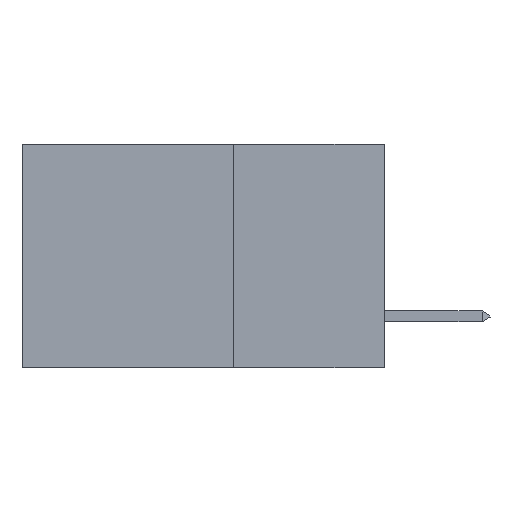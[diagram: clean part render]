
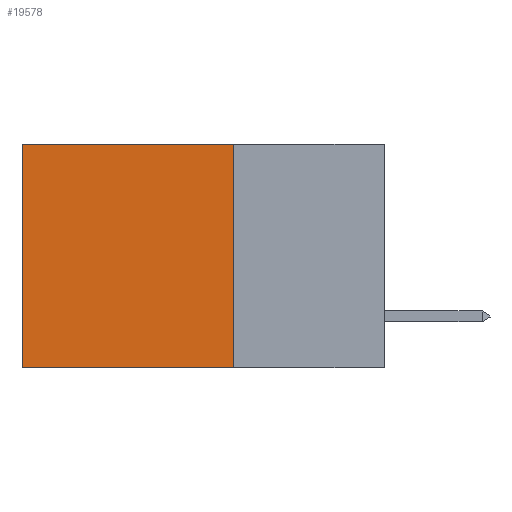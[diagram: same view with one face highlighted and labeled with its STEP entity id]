
A CAD part, left-side view. The second image highlights one B-rep face of the part: STEP entity #19578.
In plain terms, the highlighted planar face has unit normal (-1, 0, 0).
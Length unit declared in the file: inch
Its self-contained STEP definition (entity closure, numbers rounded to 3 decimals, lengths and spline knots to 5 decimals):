
#1163 = CARTESIAN_POINT ( 'NONE',  ( 0.2875, 0.6, 0. ) ) ;
#6717 = VERTEX_POINT ( 'NONE', #48177 ) ;
#6965 = CARTESIAN_POINT ( 'NONE',  ( 0.2875, 0.25, 0. ) ) ;
#9859 = CARTESIAN_POINT ( 'NONE',  ( 0.2875, 0.6, 0. ) ) ;
#10249 = EDGE_CURVE ( 'NONE', #44235, #6717, #15977, .T. ) ;
#10529 = EDGE_LOOP ( 'NONE', ( #20024, #29664, #13233, #15975 ) ) ;
#11684 = CARTESIAN_POINT ( 'NONE',  ( 0.2875, 0.25, -0.37 ) ) ;
#13233 = ORIENTED_EDGE ( 'NONE', *, *, #30695, .F. ) ;
#13347 = CARTESIAN_POINT ( 'NONE',  ( 0.2875, 0.25, -0.37 ) ) ;
#13604 = LINE ( 'NONE', #26732, #15287 ) ;
#15287 = VECTOR ( 'NONE', #26277, 39.37008 ) ;
#15975 = ORIENTED_EDGE ( 'NONE', *, *, #32435, .T. ) ;
#15977 = LINE ( 'NONE', #1163, #42293 ) ;
#19578 = ADVANCED_FACE ( 'NONE', ( #25857 ), #25882, .F. ) ;
#20024 = ORIENTED_EDGE ( 'NONE', *, *, #10249, .T. ) ;
#21799 = DIRECTION ( 'NONE',  ( 1., 0., 0. ) ) ;
#21979 = LINE ( 'NONE', #11684, #39513 ) ;
#23396 = VERTEX_POINT ( 'NONE', #13347 ) ;
#25857 = FACE_OUTER_BOUND ( 'NONE', #10529, .T. ) ;
#25882 = PLANE ( 'NONE',  #27181 ) ;
#26277 = DIRECTION ( 'NONE',  ( 0., 1., 0. ) ) ;
#26732 = CARTESIAN_POINT ( 'NONE',  ( 0.2875, 0.25, 0. ) ) ;
#27181 = AXIS2_PLACEMENT_3D ( 'NONE', #6965, #21799, #44071 ) ;
#28309 = CARTESIAN_POINT ( 'NONE',  ( 0.2875, 0.25, 0. ) ) ;
#29664 = ORIENTED_EDGE ( 'NONE', *, *, #30523, .F. ) ;
#30523 = EDGE_CURVE ( 'NONE', #23396, #6717, #21979, .T. ) ;
#30695 = EDGE_CURVE ( 'NONE', #43369, #23396, #47689, .T. ) ;
#32435 = EDGE_CURVE ( 'NONE', #43369, #44235, #13604, .T. ) ;
#34197 = DIRECTION ( 'NONE',  ( 0., 1., 0. ) ) ;
#37729 = VECTOR ( 'NONE', #44540, 39.37008 ) ;
#39513 = VECTOR ( 'NONE', #34197, 39.37008 ) ;
#40646 = CARTESIAN_POINT ( 'NONE',  ( 0.2875, 0.25, 0. ) ) ;
#42293 = VECTOR ( 'NONE', #46274, 39.37008 ) ;
#43369 = VERTEX_POINT ( 'NONE', #40646 ) ;
#44071 = DIRECTION ( 'NONE',  ( 0., 0., -1. ) ) ;
#44235 = VERTEX_POINT ( 'NONE', #9859 ) ;
#44540 = DIRECTION ( 'NONE',  ( 0., 0., -1. ) ) ;
#46274 = DIRECTION ( 'NONE',  ( 0., 0., -1. ) ) ;
#47689 = LINE ( 'NONE', #28309, #37729 ) ;
#48177 = CARTESIAN_POINT ( 'NONE',  ( 0.2875, 0.6, -0.37 ) ) ;
